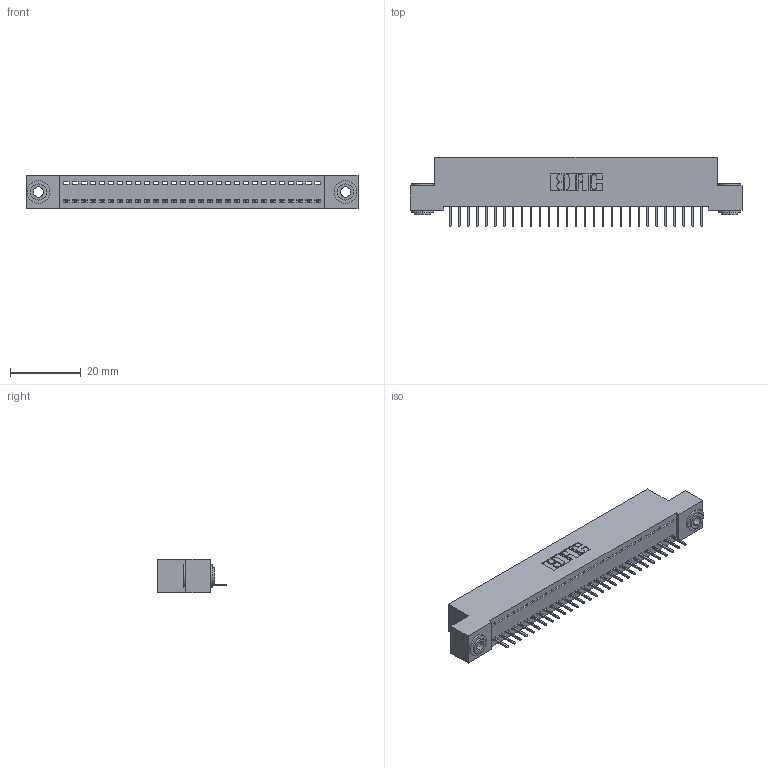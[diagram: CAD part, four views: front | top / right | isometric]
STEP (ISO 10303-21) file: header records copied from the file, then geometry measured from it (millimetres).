
FILE_DESCRIPTION (( 'STEP AP203' ), '1' );
FILE_NAME ('342-029-524-103.STEP', '2019-10-02T03:45:05', ( '' ), ( '' ), 'SwSTEP 2.0', 'SolidWorks 2016', '' );
FILE_SCHEMA (( 'CONFIG_CONTROL_DESIGN' ));
Length unit declared in the file: inch
Products named in the file (4): 342 Part_.156 TH; 345-292-001_345-293-124; 342-250-002_345-250-002-102; 342-029-524-103
Assembly tree (32 placements, depth 2):
  342-029-524-103
    342 Part_.156 TH
    345-292-001_345-293-124  x29
    342-250-002_345-250-002-102  x2
Bounding box: 93.98 x 19.69 x 9.4 mm (x, y, z)
Volume: 8100.5 mm3; surface area: 11522.9 mm2
Topology: 32 solids, 32 shells, 1946 faces, 5595 edges, 3610 vertices
Faces by surface type: plane 1468, cylinder 470, cone 8
Entity records: 20002 total; most frequent: CARTESIAN_POINT 3428, ORIENTED_EDGE 3386, DIRECTION 2953, EDGE_CURVE 1693, VECTOR 1545, LINE 1545, VERTEX_POINT 1122, AXIS2_PLACEMENT_3D 704
